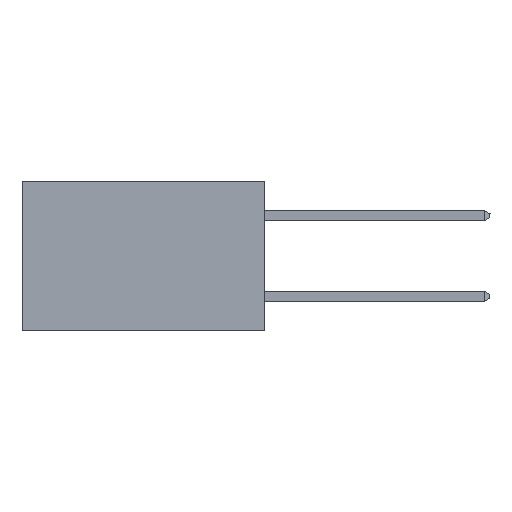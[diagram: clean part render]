
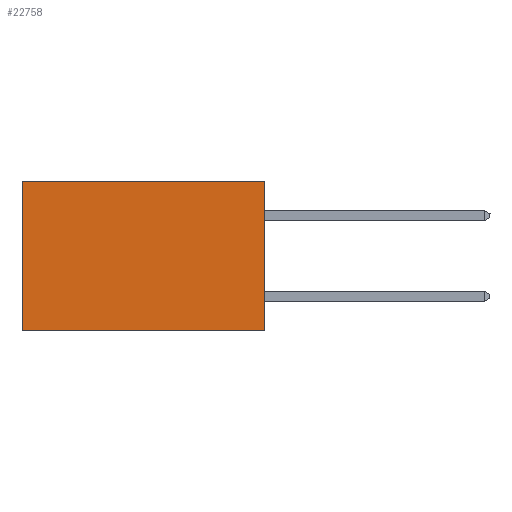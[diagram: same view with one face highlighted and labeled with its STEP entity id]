
A CAD part, left-side view. The second image highlights one B-rep face of the part: STEP entity #22758.
In plain terms, the highlighted planar face has unit normal (-1, 0, 0).
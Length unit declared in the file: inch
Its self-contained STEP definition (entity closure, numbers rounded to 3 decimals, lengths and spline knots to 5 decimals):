
#1185 = VERTEX_POINT ( 'NONE', #23278 ) ;
#2549 = CARTESIAN_POINT ( 'NONE',  ( 0.298, 0.6, 0. ) ) ;
#3224 = CARTESIAN_POINT ( 'NONE',  ( 0.298, 0., 0. ) ) ;
#5374 = VERTEX_POINT ( 'NONE', #8828 ) ;
#5440 = DIRECTION ( 'NONE',  ( 0., 1., 0. ) ) ;
#5774 = PLANE ( 'NONE',  #6926 ) ;
#6880 = LINE ( 'NONE', #11495, #8622 ) ;
#6926 = AXIS2_PLACEMENT_3D ( 'NONE', #9729, #9651, #7920 ) ;
#7920 = DIRECTION ( 'NONE',  ( 0., 0., -1. ) ) ;
#8070 = CARTESIAN_POINT ( 'NONE',  ( 0.298, 0., 0. ) ) ;
#8207 = ORIENTED_EDGE ( 'NONE', *, *, #11718, .T. ) ;
#8244 = EDGE_CURVE ( 'NONE', #1185, #5374, #10438, .T. ) ;
#8514 = CARTESIAN_POINT ( 'NONE',  ( 0.298, 0., -0.37 ) ) ;
#8622 = VECTOR ( 'NONE', #5440, 39.37008 ) ;
#8828 = CARTESIAN_POINT ( 'NONE',  ( 0.298, 0.6, -0.37 ) ) ;
#8867 = FACE_OUTER_BOUND ( 'NONE', #21682, .T. ) ;
#9651 = DIRECTION ( 'NONE',  ( 1., 0., 0. ) ) ;
#9729 = CARTESIAN_POINT ( 'NONE',  ( 0.298, 0., 0. ) ) ;
#10438 = LINE ( 'NONE', #2549, #14207 ) ;
#11188 = ORIENTED_EDGE ( 'NONE', *, *, #8244, .T. ) ;
#11495 = CARTESIAN_POINT ( 'NONE',  ( 0.298, 0., -0.37 ) ) ;
#11718 = EDGE_CURVE ( 'NONE', #18266, #1185, #17300, .T. ) ;
#12396 = VECTOR ( 'NONE', #13513, 39.37008 ) ;
#13513 = DIRECTION ( 'NONE',  ( 0., 1., 0. ) ) ;
#13860 = ORIENTED_EDGE ( 'NONE', *, *, #21874, .F. ) ;
#14044 = CARTESIAN_POINT ( 'NONE',  ( 0.298, 0., 0. ) ) ;
#14207 = VECTOR ( 'NONE', #17249, 39.37008 ) ;
#15091 = VERTEX_POINT ( 'NONE', #8514 ) ;
#17249 = DIRECTION ( 'NONE',  ( 0., 0., -1. ) ) ;
#17300 = LINE ( 'NONE', #8070, #12396 ) ;
#18237 = EDGE_CURVE ( 'NONE', #18266, #15091, #20948, .T. ) ;
#18266 = VERTEX_POINT ( 'NONE', #3224 ) ;
#20948 = LINE ( 'NONE', #14044, #21542 ) ;
#21462 = DIRECTION ( 'NONE',  ( 0., 0., -1. ) ) ;
#21542 = VECTOR ( 'NONE', #21462, 39.37008 ) ;
#21682 = EDGE_LOOP ( 'NONE', ( #11188, #13860, #21785, #8207 ) ) ;
#21785 = ORIENTED_EDGE ( 'NONE', *, *, #18237, .F. ) ;
#21874 = EDGE_CURVE ( 'NONE', #15091, #5374, #6880, .T. ) ;
#22758 = ADVANCED_FACE ( 'NONE', ( #8867 ), #5774, .F. ) ;
#23278 = CARTESIAN_POINT ( 'NONE',  ( 0.298, 0.6, 0. ) ) ;
